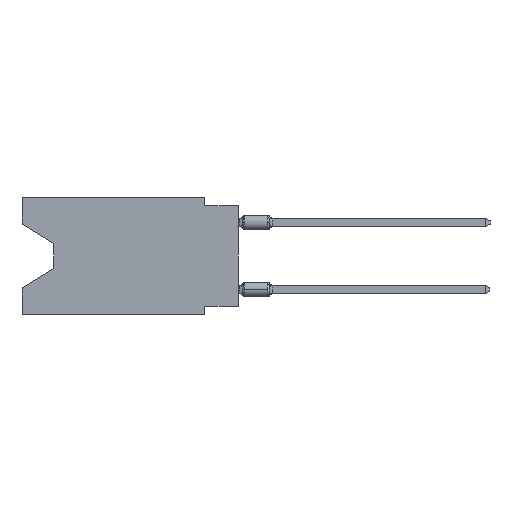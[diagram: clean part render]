
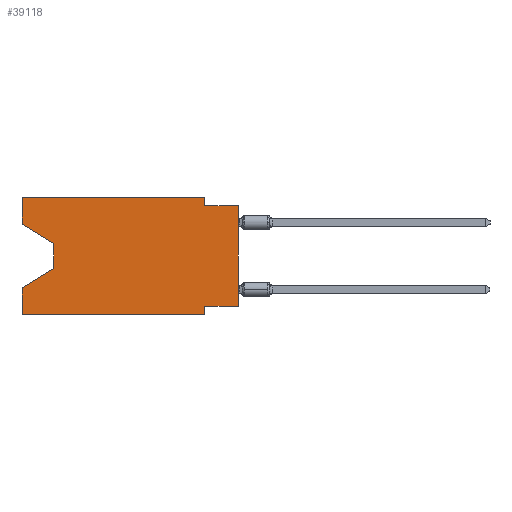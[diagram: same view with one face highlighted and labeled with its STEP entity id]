
A CAD part, left-side view. The second image highlights one B-rep face of the part: STEP entity #39118.
In plain terms, the highlighted planar face has unit normal (-1, 0, 0).
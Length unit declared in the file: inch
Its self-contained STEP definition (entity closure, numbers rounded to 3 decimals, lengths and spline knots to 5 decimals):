
#371 = ORIENTED_EDGE ( 'NONE', *, *, #11577, .F. ) ;
#840 = CARTESIAN_POINT ( 'NONE',  ( 0., 0.645, -0.35 ) ) ;
#1111 = EDGE_CURVE ( 'NONE', #32018, #44531, #20937, .T. ) ;
#1656 = VERTEX_POINT ( 'NONE', #12116 ) ;
#2530 = ORIENTED_EDGE ( 'NONE', *, *, #35767, .T. ) ;
#2825 = CARTESIAN_POINT ( 'NONE',  ( 0., 0.1, -0.025 ) ) ;
#3212 = EDGE_CURVE ( 'NONE', #29130, #13424, #7180, .T. ) ;
#3379 = LINE ( 'NONE', #16659, #11131 ) ;
#4546 = CARTESIAN_POINT ( 'NONE',  ( 0., 0., -0.325 ) ) ;
#4876 = EDGE_CURVE ( 'NONE', #42602, #36873, #31974, .T. ) ;
#5266 = CARTESIAN_POINT ( 'NONE',  ( 0., 0.645, 0. ) ) ;
#5350 = ORIENTED_EDGE ( 'NONE', *, *, #34676, .T. ) ;
#5563 = VERTEX_POINT ( 'NONE', #2825 ) ;
#6003 = DIRECTION ( 'NONE',  ( 0., 0., 1. ) ) ;
#7075 = VECTOR ( 'NONE', #40708, 39.37008 ) ;
#7180 = LINE ( 'NONE', #27793, #33294 ) ;
#7211 = EDGE_CURVE ( 'NONE', #5563, #36018, #37998, .T. ) ;
#7566 = LINE ( 'NONE', #42370, #30574 ) ;
#7752 = VERTEX_POINT ( 'NONE', #39297 ) ;
#7837 = CARTESIAN_POINT ( 'NONE',  ( 0., 0.645, 0. ) ) ;
#11131 = VECTOR ( 'NONE', #37943, 39.37008 ) ;
#11455 = EDGE_CURVE ( 'NONE', #33325, #1656, #3379, .T. ) ;
#11577 = EDGE_CURVE ( 'NONE', #13424, #36873, #18004, .T. ) ;
#11677 = DIRECTION ( 'NONE',  ( 0., -0.855, -0.519 ) ) ;
#12032 = CARTESIAN_POINT ( 'NONE',  ( 0., 0.1, -0.35 ) ) ;
#12116 = CARTESIAN_POINT ( 'NONE',  ( 0., 0.55, -0.212 ) ) ;
#12541 = DIRECTION ( 'NONE',  ( 0., 0.855, -0.519 ) ) ;
#12808 = ORIENTED_EDGE ( 'NONE', *, *, #23085, .F. ) ;
#12957 = ORIENTED_EDGE ( 'NONE', *, *, #4876, .T. ) ;
#13424 = VERTEX_POINT ( 'NONE', #30528 ) ;
#14320 = DIRECTION ( 'NONE',  ( 0., 0., 1. ) ) ;
#14802 = CARTESIAN_POINT ( 'NONE',  ( 0., 0.645, 0. ) ) ;
#14830 = CARTESIAN_POINT ( 'NONE',  ( 0., 0.1, -0.35 ) ) ;
#15993 = ORIENTED_EDGE ( 'NONE', *, *, #1111, .F. ) ;
#16242 = LINE ( 'NONE', #25873, #7075 ) ;
#16659 = CARTESIAN_POINT ( 'NONE',  ( 0., 0.55, -0.138 ) ) ;
#16763 = LINE ( 'NONE', #27279, #22645 ) ;
#17909 = FACE_OUTER_BOUND ( 'NONE', #23389, .T. ) ;
#18004 = LINE ( 'NONE', #14830, #22805 ) ;
#19597 = VECTOR ( 'NONE', #34562, 39.37008 ) ;
#20602 = CARTESIAN_POINT ( 'NONE',  ( 0., 0., -0.025 ) ) ;
#20727 = CARTESIAN_POINT ( 'NONE',  ( 0., 0.645, 0. ) ) ;
#20937 = LINE ( 'NONE', #20727, #43743 ) ;
#21151 = DIRECTION ( 'NONE',  ( 0., 1., 0. ) ) ;
#21317 = VERTEX_POINT ( 'NONE', #33462 ) ;
#22414 = ORIENTED_EDGE ( 'NONE', *, *, #44456, .F. ) ;
#22645 = VECTOR ( 'NONE', #6003, 39.37008 ) ;
#22805 = VECTOR ( 'NONE', #42530, 39.37008 ) ;
#23085 = EDGE_CURVE ( 'NONE', #42602, #21317, #36640, .T. ) ;
#23243 = CARTESIAN_POINT ( 'NONE',  ( 0., 0.55, -0.138 ) ) ;
#23389 = EDGE_LOOP ( 'NONE', ( #38422, #25805, #2530, #12808, #12957, #371, #27996, #5350, #26708, #29332, #22414, #15993 ) ) ;
#25544 = CARTESIAN_POINT ( 'NONE',  ( 0., 0.645, 0. ) ) ;
#25584 = CARTESIAN_POINT ( 'NONE',  ( 0., 0.645, -0.35 ) ) ;
#25805 = ORIENTED_EDGE ( 'NONE', *, *, #11455, .T. ) ;
#25873 = CARTESIAN_POINT ( 'NONE',  ( 0., 0.1, 0. ) ) ;
#26182 = VECTOR ( 'NONE', #39854, 39.37008 ) ;
#26246 = VECTOR ( 'NONE', #35388, 39.37008 ) ;
#26708 = ORIENTED_EDGE ( 'NONE', *, *, #7211, .F. ) ;
#27097 = VECTOR ( 'NONE', #12541, 39.37008 ) ;
#27279 = CARTESIAN_POINT ( 'NONE',  ( 0., 0., 0. ) ) ;
#27793 = CARTESIAN_POINT ( 'NONE',  ( 0., 0., -0.325 ) ) ;
#27996 = ORIENTED_EDGE ( 'NONE', *, *, #3212, .F. ) ;
#28386 = VECTOR ( 'NONE', #42752, 39.37008 ) ;
#28456 = CARTESIAN_POINT ( 'NONE',  ( 0., 0., -0.025 ) ) ;
#28669 = PLANE ( 'NONE',  #39026 ) ;
#29130 = VERTEX_POINT ( 'NONE', #4546 ) ;
#29332 = ORIENTED_EDGE ( 'NONE', *, *, #41985, .F. ) ;
#30112 = CARTESIAN_POINT ( 'NONE',  ( 0., 0.645, -0.08025 ) ) ;
#30154 = LINE ( 'NONE', #34027, #27097 ) ;
#30528 = CARTESIAN_POINT ( 'NONE',  ( 0., 0.1, -0.325 ) ) ;
#30574 = VECTOR ( 'NONE', #11677, 39.37008 ) ;
#31974 = LINE ( 'NONE', #25584, #28386 ) ;
#32018 = VERTEX_POINT ( 'NONE', #30112 ) ;
#33294 = VECTOR ( 'NONE', #21151, 39.37008 ) ;
#33325 = VERTEX_POINT ( 'NONE', #23243 ) ;
#33462 = CARTESIAN_POINT ( 'NONE',  ( 0., 0.645, -0.26975 ) ) ;
#34027 = CARTESIAN_POINT ( 'NONE',  ( 0., 0.55, -0.212 ) ) ;
#34562 = DIRECTION ( 'NONE',  ( 0., -1., 0. ) ) ;
#34676 = EDGE_CURVE ( 'NONE', #29130, #36018, #16763, .T. ) ;
#35388 = DIRECTION ( 'NONE',  ( 0., -1., 0. ) ) ;
#35767 = EDGE_CURVE ( 'NONE', #1656, #21317, #30154, .T. ) ;
#36018 = VERTEX_POINT ( 'NONE', #28456 ) ;
#36640 = LINE ( 'NONE', #5266, #26182 ) ;
#36873 = VERTEX_POINT ( 'NONE', #12032 ) ;
#37943 = DIRECTION ( 'NONE',  ( 0., 0., -1. ) ) ;
#37970 = LINE ( 'NONE', #25544, #26246 ) ;
#37998 = LINE ( 'NONE', #20602, #19597 ) ;
#38422 = ORIENTED_EDGE ( 'NONE', *, *, #41867, .T. ) ;
#38509 = DIRECTION ( 'NONE',  ( 1., 0., 0. ) ) ;
#38744 = DIRECTION ( 'NONE',  ( 0., 0., -1. ) ) ;
#39026 = AXIS2_PLACEMENT_3D ( 'NONE', #7837, #38509, #38744 ) ;
#39118 = ADVANCED_FACE ( 'NONE', ( #17909 ), #28669, .F. ) ;
#39297 = CARTESIAN_POINT ( 'NONE',  ( 0., 0.1, 0. ) ) ;
#39854 = DIRECTION ( 'NONE',  ( 0., 0., 1. ) ) ;
#40708 = DIRECTION ( 'NONE',  ( 0., 0., -1. ) ) ;
#41867 = EDGE_CURVE ( 'NONE', #32018, #33325, #7566, .T. ) ;
#41985 = EDGE_CURVE ( 'NONE', #7752, #5563, #16242, .T. ) ;
#42370 = CARTESIAN_POINT ( 'NONE',  ( 0., 0.645, -0.08025 ) ) ;
#42530 = DIRECTION ( 'NONE',  ( 0., 0., -1. ) ) ;
#42602 = VERTEX_POINT ( 'NONE', #840 ) ;
#42752 = DIRECTION ( 'NONE',  ( 0., -1., 0. ) ) ;
#43743 = VECTOR ( 'NONE', #14320, 39.37008 ) ;
#44456 = EDGE_CURVE ( 'NONE', #44531, #7752, #37970, .T. ) ;
#44531 = VERTEX_POINT ( 'NONE', #14802 ) ;
